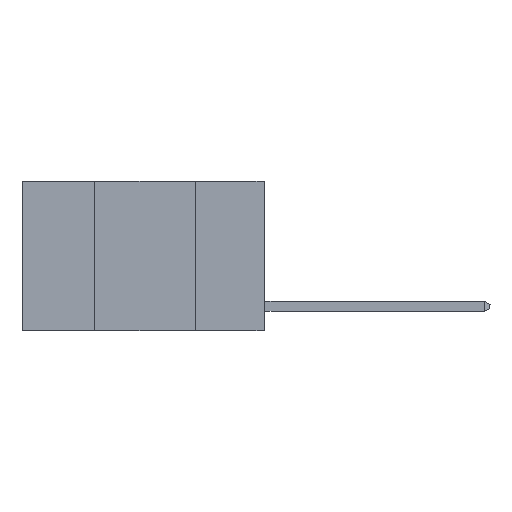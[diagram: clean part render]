
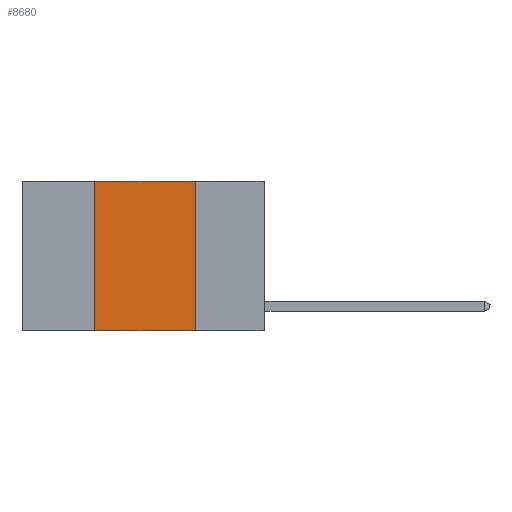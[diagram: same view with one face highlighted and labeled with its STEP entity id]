
A CAD part, left-side view. The second image highlights one B-rep face of the part: STEP entity #8680.
In plain terms, the highlighted planar face has unit normal (-1, 0, 0).
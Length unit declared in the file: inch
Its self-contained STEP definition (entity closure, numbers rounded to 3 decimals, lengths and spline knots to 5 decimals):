
#225 = ORIENTED_EDGE ( 'NONE', *, *, #2862, .F. ) ;
#276 = ORIENTED_EDGE ( 'NONE', *, *, #9563, .F. ) ;
#389 = ORIENTED_EDGE ( 'NONE', *, *, #10364, .F. ) ;
#398 = VECTOR ( 'NONE', #4228, 39.37008 ) ;
#431 = ORIENTED_EDGE ( 'NONE', *, *, #9375, .T. ) ;
#1605 = CARTESIAN_POINT ( 'NONE',  ( 0., 0.17, 0. ) ) ;
#1905 = DIRECTION ( 'NONE',  ( 0., 0., 1. ) ) ;
#2649 = VERTEX_POINT ( 'NONE', #5685 ) ;
#2862 = EDGE_CURVE ( 'NONE', #10774, #4205, #5354, .T. ) ;
#3486 = LINE ( 'NONE', #9479, #8240 ) ;
#3579 = DIRECTION ( 'NONE',  ( 0., 0., -1. ) ) ;
#3620 = CARTESIAN_POINT ( 'NONE',  ( 0., 0.17, 0. ) ) ;
#4205 = VERTEX_POINT ( 'NONE', #6016 ) ;
#4228 = DIRECTION ( 'NONE',  ( 0., -1., 0. ) ) ;
#4445 = VERTEX_POINT ( 'NONE', #10171 ) ;
#4591 = CARTESIAN_POINT ( 'NONE',  ( 0., 0.6, 0. ) ) ;
#5354 = LINE ( 'NONE', #3620, #7575 ) ;
#5545 = DIRECTION ( 'NONE',  ( 0., 0., -1. ) ) ;
#5615 = LINE ( 'NONE', #7286, #5916 ) ;
#5685 = CARTESIAN_POINT ( 'NONE',  ( 0., 0.42, -0.37 ) ) ;
#5916 = VECTOR ( 'NONE', #10993, 39.37008 ) ;
#6016 = CARTESIAN_POINT ( 'NONE',  ( 0., 0.17, -0.37 ) ) ;
#6860 = AXIS2_PLACEMENT_3D ( 'NONE', #4591, #11133, #5545 ) ;
#6965 = EDGE_LOOP ( 'NONE', ( #225, #276, #389, #431 ) ) ;
#7286 = CARTESIAN_POINT ( 'NONE',  ( 0., 0.6, 0. ) ) ;
#7575 = VECTOR ( 'NONE', #3579, 39.37008 ) ;
#8240 = VECTOR ( 'NONE', #1905, 39.37008 ) ;
#8680 = ADVANCED_FACE ( 'NONE', ( #10333 ), #9284, .F. ) ;
#9284 = PLANE ( 'NONE',  #6860 ) ;
#9375 = EDGE_CURVE ( 'NONE', #2649, #4205, #9884, .T. ) ;
#9479 = CARTESIAN_POINT ( 'NONE',  ( 0., 0.42, 0. ) ) ;
#9563 = EDGE_CURVE ( 'NONE', #4445, #10774, #5615, .T. ) ;
#9874 = CARTESIAN_POINT ( 'NONE',  ( 0., 0.6, -0.37 ) ) ;
#9884 = LINE ( 'NONE', #9874, #398 ) ;
#10171 = CARTESIAN_POINT ( 'NONE',  ( 0., 0.42, 0. ) ) ;
#10333 = FACE_OUTER_BOUND ( 'NONE', #6965, .T. ) ;
#10364 = EDGE_CURVE ( 'NONE', #2649, #4445, #3486, .T. ) ;
#10774 = VERTEX_POINT ( 'NONE', #1605 ) ;
#10993 = DIRECTION ( 'NONE',  ( 0., -1., 0. ) ) ;
#11133 = DIRECTION ( 'NONE',  ( 1., 0., 0. ) ) ;
